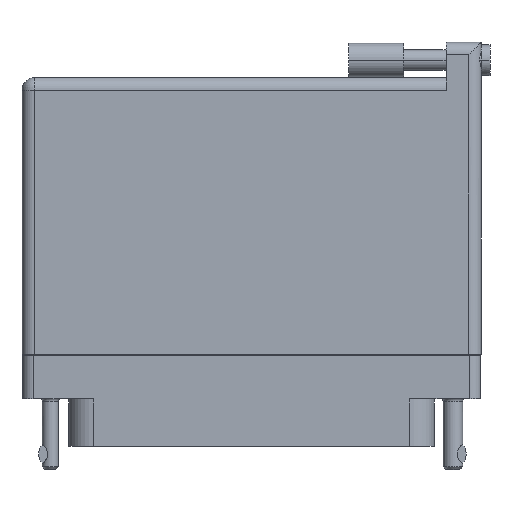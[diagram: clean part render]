
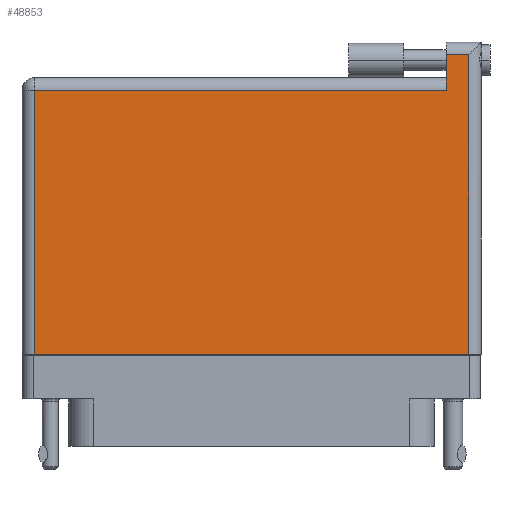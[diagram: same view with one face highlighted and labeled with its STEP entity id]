
A CAD part, front view. The second image highlights one B-rep face of the part: STEP entity #48853.
In plain terms, the highlighted face is planar.
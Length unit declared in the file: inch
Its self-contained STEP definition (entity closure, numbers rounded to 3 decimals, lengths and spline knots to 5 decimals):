
#839 = CARTESIAN_POINT ( 'NONE',  ( -1.3, 1.596, 0.4495 ) ) ;
#2617 = VECTOR ( 'NONE', #26926, 39.37008 ) ;
#3384 = FACE_OUTER_BOUND ( 'NONE', #41422, .T. ) ;
#7956 = EDGE_CURVE ( 'NONE', #48038, #39716, #51912, .T. ) ;
#8073 = VERTEX_POINT ( 'NONE', #37421 ) ;
#8882 = VECTOR ( 'NONE', #36056, 39.37008 ) ;
#9500 = EDGE_CURVE ( 'NONE', #8073, #20246, #46406, .T. ) ;
#11398 = ORIENTED_EDGE ( 'NONE', *, *, #9500, .T. ) ;
#11803 = LINE ( 'NONE', #34820, #44910 ) ;
#12341 = DIRECTION ( 'NONE',  ( 0., 0., -1. ) ) ;
#13829 = ORIENTED_EDGE ( 'NONE', *, *, #41538, .T. ) ;
#15314 = LINE ( 'NONE', #56485, #42624 ) ;
#16298 = EDGE_CURVE ( 'NONE', #24544, #8073, #11803, .T. ) ;
#17690 = AXIS2_PLACEMENT_3D ( 'NONE', #40723, #12341, #45233 ) ;
#19827 = VECTOR ( 'NONE', #52043, 39.37008 ) ;
#19959 = DIRECTION ( 'NONE',  ( 0., -1., 0. ) ) ;
#20246 = VERTEX_POINT ( 'NONE', #39195 ) ;
#21518 = LINE ( 'NONE', #29426, #57517 ) ;
#21550 = ORIENTED_EDGE ( 'NONE', *, *, #16298, .T. ) ;
#22043 = LINE ( 'NONE', #839, #19827 ) ;
#24544 = VERTEX_POINT ( 'NONE', #40724 ) ;
#25669 = CARTESIAN_POINT ( 'NONE',  ( 1.23, -0.1, 0.4495 ) ) ;
#26926 = DIRECTION ( 'NONE',  ( 0., 1., 0. ) ) ;
#27541 = VERTEX_POINT ( 'NONE', #49388 ) ;
#29426 = CARTESIAN_POINT ( 'NONE',  ( -1.3, -0.1, 0.4495 ) ) ;
#34820 = CARTESIAN_POINT ( 'NONE',  ( 1.103, 1.666, 0.4495 ) ) ;
#35828 = PLANE ( 'NONE',  #17690 ) ;
#36056 = DIRECTION ( 'NONE',  ( -1., 0., 0. ) ) ;
#36512 = CARTESIAN_POINT ( 'NONE',  ( 1.23, 1.596, 0.4495 ) ) ;
#37421 = CARTESIAN_POINT ( 'NONE',  ( 1.103, 1.396, 0.4495 ) ) ;
#39195 = CARTESIAN_POINT ( 'NONE',  ( -1.23, 1.396, 0.4495 ) ) ;
#39716 = VERTEX_POINT ( 'NONE', #36512 ) ;
#40723 = CARTESIAN_POINT ( 'NONE',  ( -1.3, 1.466, 0.4495 ) ) ;
#40724 = CARTESIAN_POINT ( 'NONE',  ( 1.103, 1.596, 0.4495 ) ) ;
#41422 = EDGE_LOOP ( 'NONE', ( #13829, #56159, #56228, #21550, #11398, #58297 ) ) ;
#41538 = EDGE_CURVE ( 'NONE', #27541, #48038, #21518, .T. ) ;
#42444 = DIRECTION ( 'NONE',  ( 0., -1., 0. ) ) ;
#42624 = VECTOR ( 'NONE', #42444, 39.37008 ) ;
#44910 = VECTOR ( 'NONE', #19959, 39.37008 ) ;
#45233 = DIRECTION ( 'NONE',  ( -1., 0., 0. ) ) ;
#45613 = CARTESIAN_POINT ( 'NONE',  ( 1.23, 1.666, 0.4495 ) ) ;
#46406 = LINE ( 'NONE', #59919, #8882 ) ;
#47527 = EDGE_CURVE ( 'NONE', #20246, #27541, #15314, .T. ) ;
#48038 = VERTEX_POINT ( 'NONE', #25669 ) ;
#48853 = ADVANCED_FACE ( 'NONE', ( #3384 ), #35828, .F. ) ;
#49388 = CARTESIAN_POINT ( 'NONE',  ( -1.23, -0.1, 0.4495 ) ) ;
#51912 = LINE ( 'NONE', #45613, #2617 ) ;
#52043 = DIRECTION ( 'NONE',  ( -1., 0., 0. ) ) ;
#56159 = ORIENTED_EDGE ( 'NONE', *, *, #7956, .T. ) ;
#56228 = ORIENTED_EDGE ( 'NONE', *, *, #59497, .T. ) ;
#56485 = CARTESIAN_POINT ( 'NONE',  ( -1.23, -0.1, 0.4495 ) ) ;
#57517 = VECTOR ( 'NONE', #57648, 39.37008 ) ;
#57648 = DIRECTION ( 'NONE',  ( 1., 0., 0. ) ) ;
#58297 = ORIENTED_EDGE ( 'NONE', *, *, #47527, .T. ) ;
#59497 = EDGE_CURVE ( 'NONE', #39716, #24544, #22043, .T. ) ;
#59919 = CARTESIAN_POINT ( 'NONE',  ( -1.3, 1.396, 0.4495 ) ) ;
